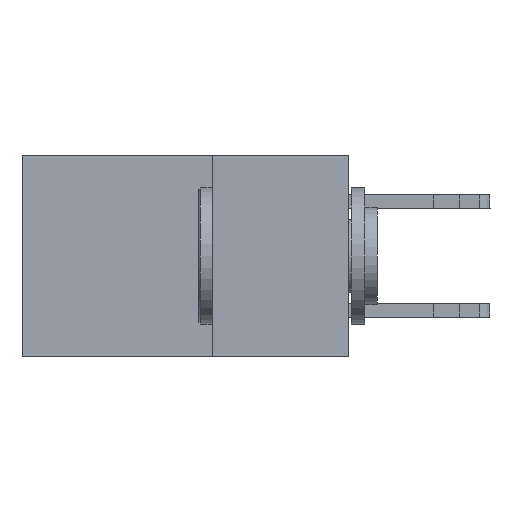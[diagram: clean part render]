
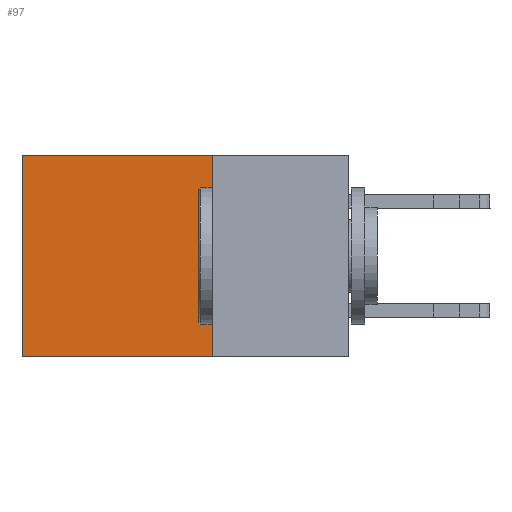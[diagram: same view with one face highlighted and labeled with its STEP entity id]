
A CAD part, left-side view. The second image highlights one B-rep face of the part: STEP entity #97.
In plain terms, the highlighted planar face has unit normal (-1, 0, 0).
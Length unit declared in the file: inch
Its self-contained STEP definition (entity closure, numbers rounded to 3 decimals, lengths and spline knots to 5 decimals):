
#97 = ADVANCED_FACE ( 'NONE', ( #10562 ), #384, .F. ) ;
#320 = CARTESIAN_POINT ( 'NONE',  ( 0.298, 0.25, 0. ) ) ;
#384 = PLANE ( 'NONE',  #6568 ) ;
#484 = ORIENTED_EDGE ( 'NONE', *, *, #3066, .T. ) ;
#1134 = LINE ( 'NONE', #8244, #11062 ) ;
#1250 = LINE ( 'NONE', #4305, #5747 ) ;
#1348 = EDGE_CURVE ( 'NONE', #3386, #9406, #5049, .T. ) ;
#1557 = DIRECTION ( 'NONE',  ( 0., 1., 0. ) ) ;
#1944 = DIRECTION ( 'NONE',  ( 0., 1., 0. ) ) ;
#2008 = CARTESIAN_POINT ( 'NONE',  ( 0.298, 0.6, 0. ) ) ;
#2549 = CARTESIAN_POINT ( 'NONE',  ( 0.298, 0.25, 0. ) ) ;
#3066 = EDGE_CURVE ( 'NONE', #12560, #7912, #11662, .T. ) ;
#3386 = VERTEX_POINT ( 'NONE', #4650 ) ;
#4305 = CARTESIAN_POINT ( 'NONE',  ( 0.298, 0.6, 0. ) ) ;
#4441 = DIRECTION ( 'NONE',  ( 0., 0., -1. ) ) ;
#4650 = CARTESIAN_POINT ( 'NONE',  ( 0.298, 0.25, -0.37 ) ) ;
#5049 = LINE ( 'NONE', #9115, #5600 ) ;
#5187 = DIRECTION ( 'NONE',  ( 0., 0., -1. ) ) ;
#5266 = CARTESIAN_POINT ( 'NONE',  ( 0.298, 0.6, -0.37 ) ) ;
#5317 = DIRECTION ( 'NONE',  ( 0., 0., -1. ) ) ;
#5600 = VECTOR ( 'NONE', #1944, 39.37008 ) ;
#5747 = VECTOR ( 'NONE', #5317, 39.37008 ) ;
#6568 = AXIS2_PLACEMENT_3D ( 'NONE', #320, #11492, #4441 ) ;
#6583 = ORIENTED_EDGE ( 'NONE', *, *, #1348, .F. ) ;
#7141 = VECTOR ( 'NONE', #1557, 39.37008 ) ;
#7912 = VERTEX_POINT ( 'NONE', #2008 ) ;
#8244 = CARTESIAN_POINT ( 'NONE',  ( 0.298, 0.25, 0. ) ) ;
#8445 = EDGE_CURVE ( 'NONE', #7912, #9406, #1250, .T. ) ;
#9115 = CARTESIAN_POINT ( 'NONE',  ( 0.298, 0.25, -0.37 ) ) ;
#9406 = VERTEX_POINT ( 'NONE', #5266 ) ;
#9838 = ORIENTED_EDGE ( 'NONE', *, *, #8445, .T. ) ;
#9854 = EDGE_CURVE ( 'NONE', #12560, #3386, #1134, .T. ) ;
#10562 = FACE_OUTER_BOUND ( 'NONE', #10737, .T. ) ;
#10737 = EDGE_LOOP ( 'NONE', ( #9838, #6583, #11034, #484 ) ) ;
#11034 = ORIENTED_EDGE ( 'NONE', *, *, #9854, .F. ) ;
#11062 = VECTOR ( 'NONE', #5187, 39.37008 ) ;
#11194 = CARTESIAN_POINT ( 'NONE',  ( 0.298, 0.25, 0. ) ) ;
#11492 = DIRECTION ( 'NONE',  ( 1., 0., 0. ) ) ;
#11662 = LINE ( 'NONE', #2549, #7141 ) ;
#12560 = VERTEX_POINT ( 'NONE', #11194 ) ;
